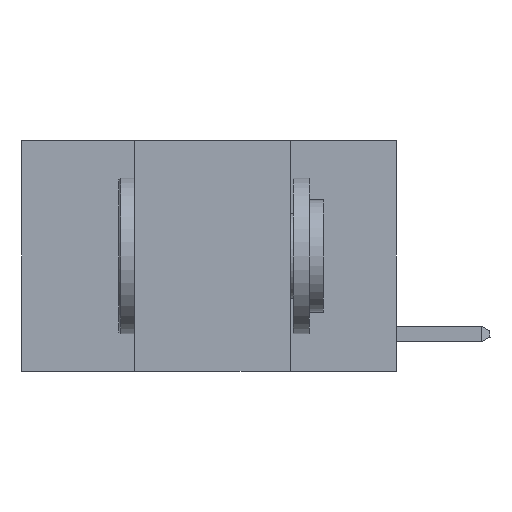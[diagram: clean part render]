
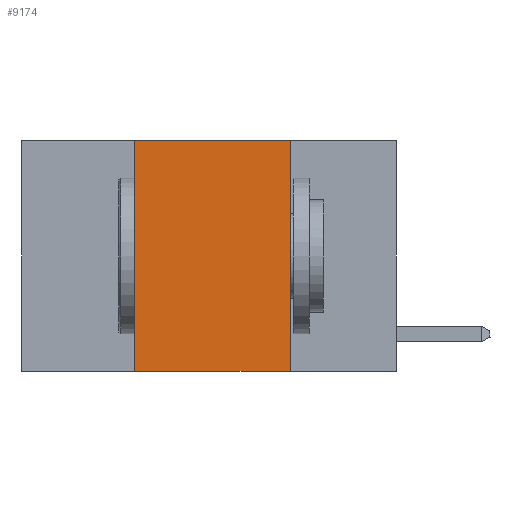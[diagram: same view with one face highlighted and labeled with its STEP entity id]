
A CAD part, left-side view. The second image highlights one B-rep face of the part: STEP entity #9174.
In plain terms, the highlighted planar face has unit normal (-1, 0, 0).
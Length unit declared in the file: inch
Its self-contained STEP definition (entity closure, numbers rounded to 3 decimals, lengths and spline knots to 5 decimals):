
#11 = CARTESIAN_POINT ( 'NONE',  ( 0., 0.42, 0. ) ) ;
#198 = VECTOR ( 'NONE', #7534, 39.37008 ) ;
#409 = VERTEX_POINT ( 'NONE', #6996 ) ;
#749 = EDGE_CURVE ( 'NONE', #9853, #409, #11524, .T. ) ;
#1012 = VERTEX_POINT ( 'NONE', #10951 ) ;
#1146 = ORIENTED_EDGE ( 'NONE', *, *, #1224, .F. ) ;
#1224 = EDGE_CURVE ( 'NONE', #409, #1012, #3772, .T. ) ;
#1275 = EDGE_LOOP ( 'NONE', ( #4761, #1146, #4163, #10983 ) ) ;
#2156 = DIRECTION ( 'NONE',  ( 0., 0., -1. ) ) ;
#3665 = DIRECTION ( 'NONE',  ( 0., -1., 0. ) ) ;
#3772 = LINE ( 'NONE', #6540, #198 ) ;
#3921 = VECTOR ( 'NONE', #4889, 39.37008 ) ;
#4163 = ORIENTED_EDGE ( 'NONE', *, *, #749, .F. ) ;
#4318 = FACE_OUTER_BOUND ( 'NONE', #1275, .T. ) ;
#4761 = ORIENTED_EDGE ( 'NONE', *, *, #5663, .F. ) ;
#4889 = DIRECTION ( 'NONE',  ( 0., 0., 1. ) ) ;
#5254 = VERTEX_POINT ( 'NONE', #6766 ) ;
#5663 = EDGE_CURVE ( 'NONE', #1012, #5254, #9550, .T. ) ;
#6433 = LINE ( 'NONE', #8245, #7950 ) ;
#6540 = CARTESIAN_POINT ( 'NONE',  ( 0., 0.6, 0. ) ) ;
#6766 = CARTESIAN_POINT ( 'NONE',  ( 0., 0.17, -0.37 ) ) ;
#6996 = CARTESIAN_POINT ( 'NONE',  ( 0., 0.42, 0. ) ) ;
#7534 = DIRECTION ( 'NONE',  ( 0., -1., 0. ) ) ;
#7950 = VECTOR ( 'NONE', #3665, 39.37008 ) ;
#7963 = PLANE ( 'NONE',  #8361 ) ;
#8245 = CARTESIAN_POINT ( 'NONE',  ( 0., 0.6, -0.37 ) ) ;
#8361 = AXIS2_PLACEMENT_3D ( 'NONE', #8782, #11739, #2156 ) ;
#8429 = EDGE_CURVE ( 'NONE', #9853, #5254, #6433, .T. ) ;
#8782 = CARTESIAN_POINT ( 'NONE',  ( 0., 0.6, 0. ) ) ;
#9174 = ADVANCED_FACE ( 'NONE', ( #4318 ), #7963, .F. ) ;
#9515 = VECTOR ( 'NONE', #9616, 39.37008 ) ;
#9550 = LINE ( 'NONE', #10553, #9515 ) ;
#9616 = DIRECTION ( 'NONE',  ( 0., 0., -1. ) ) ;
#9853 = VERTEX_POINT ( 'NONE', #11038 ) ;
#10553 = CARTESIAN_POINT ( 'NONE',  ( 0., 0.17, 0. ) ) ;
#10951 = CARTESIAN_POINT ( 'NONE',  ( 0., 0.17, 0. ) ) ;
#10983 = ORIENTED_EDGE ( 'NONE', *, *, #8429, .T. ) ;
#11038 = CARTESIAN_POINT ( 'NONE',  ( 0., 0.42, -0.37 ) ) ;
#11524 = LINE ( 'NONE', #11, #3921 ) ;
#11739 = DIRECTION ( 'NONE',  ( 1., 0., 0. ) ) ;
